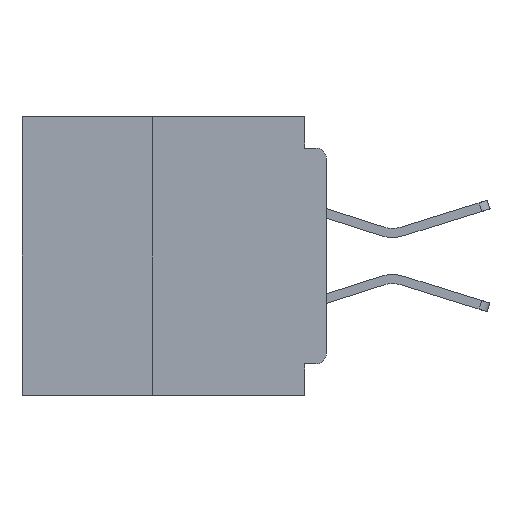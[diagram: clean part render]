
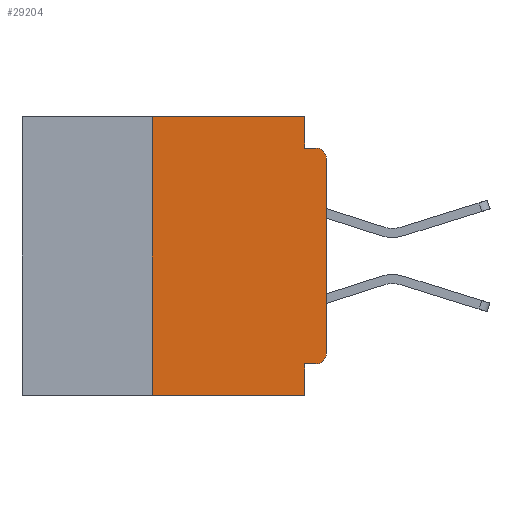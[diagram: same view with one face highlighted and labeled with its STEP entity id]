
A CAD part, left-side view. The second image highlights one B-rep face of the part: STEP entity #29204.
In plain terms, the highlighted planar face has unit normal (-1, 0, 0).
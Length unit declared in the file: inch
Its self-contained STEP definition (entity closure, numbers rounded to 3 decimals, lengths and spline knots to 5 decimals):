
#298 = ORIENTED_EDGE ( 'NONE', *, *, #15347, .F. ) ;
#472 = EDGE_CURVE ( 'NONE', #24314, #30225, #24128, .T. ) ;
#895 = DIRECTION ( 'NONE',  ( -1., 0., 0. ) ) ;
#1828 = VECTOR ( 'NONE', #31848, 39.37008 ) ;
#2369 = LINE ( 'NONE', #12934, #12322 ) ;
#2464 = VERTEX_POINT ( 'NONE', #21502 ) ;
#2931 = ORIENTED_EDGE ( 'NONE', *, *, #12505, .T. ) ;
#3015 = CIRCLE ( 'NONE', #42142, 0.015 ) ;
#3731 = CARTESIAN_POINT ( 'NONE',  ( 0., 0.015, -0.06 ) ) ;
#4128 = CARTESIAN_POINT ( 'NONE',  ( 0., 0.031, 0. ) ) ;
#4271 = ORIENTED_EDGE ( 'NONE', *, *, #472, .F. ) ;
#6679 = VECTOR ( 'NONE', #29423, 39.37008 ) ;
#6934 = VECTOR ( 'NONE', #47409, 39.37008 ) ;
#7277 = PLANE ( 'NONE',  #22344 ) ;
#7512 = CARTESIAN_POINT ( 'NONE',  ( 0., 0.015, -0.045 ) ) ;
#8021 = DIRECTION ( 'NONE',  ( 0., 0., -1. ) ) ;
#8211 = DIRECTION ( 'NONE',  ( 0., 0., -1. ) ) ;
#9667 = EDGE_CURVE ( 'NONE', #30225, #11325, #19011, .T. ) ;
#10326 = FACE_OUTER_BOUND ( 'NONE', #52792, .T. ) ;
#11325 = VERTEX_POINT ( 'NONE', #26187 ) ;
#11538 = CARTESIAN_POINT ( 'NONE',  ( 0., 0.437, 0. ) ) ;
#12322 = VECTOR ( 'NONE', #21470, 39.37008 ) ;
#12505 = EDGE_CURVE ( 'NONE', #2464, #11325, #2369, .T. ) ;
#12934 = CARTESIAN_POINT ( 'NONE',  ( 0., 0.437, -0.4 ) ) ;
#13122 = LINE ( 'NONE', #44080, #1828 ) ;
#14255 = ORIENTED_EDGE ( 'NONE', *, *, #9667, .F. ) ;
#14685 = CARTESIAN_POINT ( 'NONE',  ( 0., 0.031, -0.045 ) ) ;
#14915 = LINE ( 'NONE', #48548, #24859 ) ;
#15301 = LINE ( 'NONE', #54079, #6679 ) ;
#15347 = EDGE_CURVE ( 'NONE', #2464, #52817, #15301, .T. ) ;
#15814 = DIRECTION ( 'NONE',  ( 1., 0., 0. ) ) ;
#16394 = CARTESIAN_POINT ( 'NONE',  ( 0., 0.031, -0.4 ) ) ;
#17572 = ORIENTED_EDGE ( 'NONE', *, *, #29782, .F. ) ;
#18611 = EDGE_CURVE ( 'NONE', #24314, #34395, #3015, .T. ) ;
#19011 = LINE ( 'NONE', #16394, #27616 ) ;
#19494 = DIRECTION ( 'NONE',  ( 0., -1., 0. ) ) ;
#21132 = CARTESIAN_POINT ( 'NONE',  ( 0., 0., -0.34 ) ) ;
#21470 = DIRECTION ( 'NONE',  ( 0., -1., 0. ) ) ;
#21502 = CARTESIAN_POINT ( 'NONE',  ( 0., 0.25, -0.4 ) ) ;
#21510 = DIRECTION ( 'NONE',  ( 0., 1., 0. ) ) ;
#22063 = CARTESIAN_POINT ( 'NONE',  ( 0., 0., -0.355 ) ) ;
#22344 = AXIS2_PLACEMENT_3D ( 'NONE', #11538, #15814, #44981 ) ;
#22835 = CARTESIAN_POINT ( 'NONE',  ( 0., 0., 0. ) ) ;
#22882 = CIRCLE ( 'NONE', #50697, 0.015 ) ;
#23224 = EDGE_CURVE ( 'NONE', #34395, #37451, #31271, .T. ) ;
#23498 = ORIENTED_EDGE ( 'NONE', *, *, #23224, .T. ) ;
#24128 = LINE ( 'NONE', #22063, #44864 ) ;
#24314 = VERTEX_POINT ( 'NONE', #38345 ) ;
#24727 = CARTESIAN_POINT ( 'NONE',  ( 0., 0., -0.06 ) ) ;
#24859 = VECTOR ( 'NONE', #19494, 39.37008 ) ;
#26187 = CARTESIAN_POINT ( 'NONE',  ( 0., 0.031, -0.4 ) ) ;
#26287 = CARTESIAN_POINT ( 'NONE',  ( 0., 0.015, -0.34 ) ) ;
#26715 = EDGE_CURVE ( 'NONE', #46948, #45380, #13122, .T. ) ;
#27252 = CARTESIAN_POINT ( 'NONE',  ( 0., 0.25, 0. ) ) ;
#27616 = VECTOR ( 'NONE', #8211, 39.37008 ) ;
#28387 = EDGE_CURVE ( 'NONE', #52817, #46948, #40410, .T. ) ;
#29204 = ADVANCED_FACE ( 'NONE', ( #10326 ), #7277, .F. ) ;
#29423 = DIRECTION ( 'NONE',  ( 0., 0., 1. ) ) ;
#29782 = EDGE_CURVE ( 'NONE', #45380, #30550, #14915, .T. ) ;
#30225 = VERTEX_POINT ( 'NONE', #42922 ) ;
#30528 = DIRECTION ( 'NONE',  ( 0., 0., -1. ) ) ;
#30550 = VERTEX_POINT ( 'NONE', #7512 ) ;
#31271 = LINE ( 'NONE', #22835, #40923 ) ;
#31848 = DIRECTION ( 'NONE',  ( 0., 0., -1. ) ) ;
#32690 = ORIENTED_EDGE ( 'NONE', *, *, #28387, .F. ) ;
#33308 = DIRECTION ( 'NONE',  ( -1., 0., 0. ) ) ;
#34395 = VERTEX_POINT ( 'NONE', #21132 ) ;
#35243 = DIRECTION ( 'NONE',  ( 0., 0., 1. ) ) ;
#35444 = EDGE_CURVE ( 'NONE', #37451, #30550, #22882, .T. ) ;
#37451 = VERTEX_POINT ( 'NONE', #24727 ) ;
#38345 = CARTESIAN_POINT ( 'NONE',  ( 0., 0.015, -0.355 ) ) ;
#40410 = LINE ( 'NONE', #43259, #6934 ) ;
#40412 = ORIENTED_EDGE ( 'NONE', *, *, #18611, .T. ) ;
#40923 = VECTOR ( 'NONE', #35243, 39.37008 ) ;
#42142 = AXIS2_PLACEMENT_3D ( 'NONE', #26287, #895, #30528 ) ;
#42922 = CARTESIAN_POINT ( 'NONE',  ( 0., 0.031, -0.355 ) ) ;
#43259 = CARTESIAN_POINT ( 'NONE',  ( 0., 0.437, 0. ) ) ;
#44080 = CARTESIAN_POINT ( 'NONE',  ( 0., 0.031, 0. ) ) ;
#44864 = VECTOR ( 'NONE', #21510, 39.37008 ) ;
#44981 = DIRECTION ( 'NONE',  ( 0., 0., -1. ) ) ;
#45380 = VERTEX_POINT ( 'NONE', #14685 ) ;
#45560 = ORIENTED_EDGE ( 'NONE', *, *, #35444, .T. ) ;
#46948 = VERTEX_POINT ( 'NONE', #4128 ) ;
#47409 = DIRECTION ( 'NONE',  ( 0., -1., 0. ) ) ;
#48548 = CARTESIAN_POINT ( 'NONE',  ( 0., 0., -0.045 ) ) ;
#50697 = AXIS2_PLACEMENT_3D ( 'NONE', #3731, #33308, #8021 ) ;
#52792 = EDGE_LOOP ( 'NONE', ( #23498, #45560, #17572, #53291, #32690, #298, #2931, #14255, #4271, #40412 ) ) ;
#52817 = VERTEX_POINT ( 'NONE', #27252 ) ;
#53291 = ORIENTED_EDGE ( 'NONE', *, *, #26715, .F. ) ;
#54079 = CARTESIAN_POINT ( 'NONE',  ( 0., 0.25, -0.4 ) ) ;
